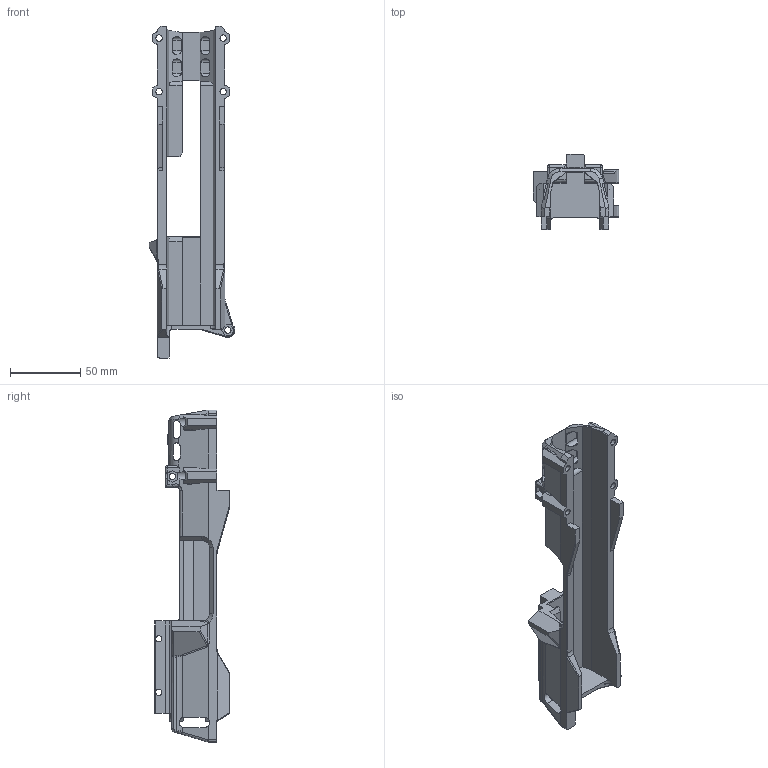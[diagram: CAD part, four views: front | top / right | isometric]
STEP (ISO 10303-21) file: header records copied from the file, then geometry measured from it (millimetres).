
FILE_DESCRIPTION (( 'STEP AP214' ), '1' );
FILE_NAME ('Hot Pocket Body.STEP', '2022-02-04T02:40:01', ( '' ), ( '' ), 'SwSTEP 2.0', 'SolidWorks 2020', '' );
FILE_SCHEMA (( 'AUTOMOTIVE_DESIGN' ));
Length unit declared in the file: inch
Products named in the file (1): Hot Pocket Body
Bounding box: 61.15 x 53.34 x 236.22 mm (x, y, z)
Volume: 108577.1 mm3; surface area: 51780.8 mm2
Topology: 1 solids, 1 shells, 397 faces, 1137 edges, 732 vertices
Faces by surface type: plane 231, cylinder 117, bspline 27, cone 18, sphere 2, torus 2
Entity records: 14267 total; most frequent: CARTESIAN_POINT 4305, ORIENTED_EDGE 2264, DIRECTION 1854, EDGE_CURVE 1132, VERTEX_POINT 732, VECTOR 732, LINE 732, AXIS2_PLACEMENT_3D 561
